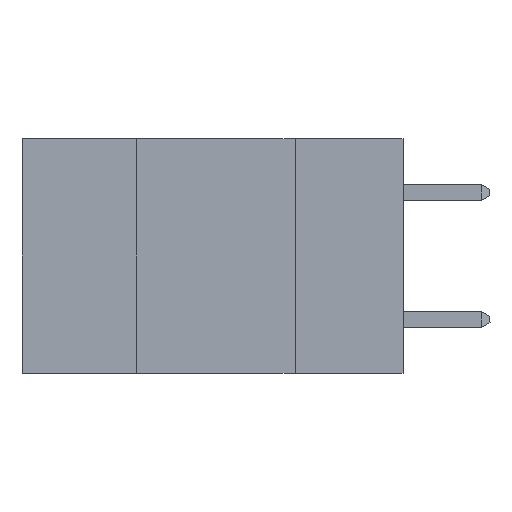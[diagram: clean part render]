
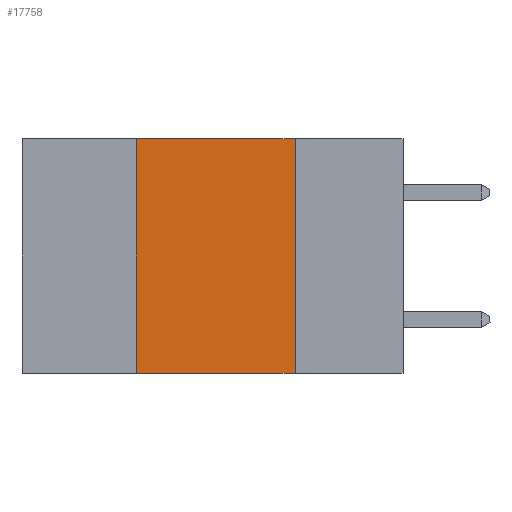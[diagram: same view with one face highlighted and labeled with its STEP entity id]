
A CAD part, left-side view. The second image highlights one B-rep face of the part: STEP entity #17758.
In plain terms, the highlighted planar face has unit normal (-1, 0, 0).
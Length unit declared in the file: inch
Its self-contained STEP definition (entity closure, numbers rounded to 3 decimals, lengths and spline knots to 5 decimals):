
#437 = CARTESIAN_POINT ( 'NONE',  ( 0., 0.42, 0. ) ) ;
#474 = VECTOR ( 'NONE', #4233, 39.37008 ) ;
#897 = EDGE_CURVE ( 'NONE', #2462, #2623, #10034, .T. ) ;
#1927 = DIRECTION ( 'NONE',  ( 0., 0., 1. ) ) ;
#2375 = VECTOR ( 'NONE', #11237, 39.37008 ) ;
#2462 = VERTEX_POINT ( 'NONE', #12152 ) ;
#2623 = VERTEX_POINT ( 'NONE', #8123 ) ;
#3463 = VERTEX_POINT ( 'NONE', #12853 ) ;
#3555 = LINE ( 'NONE', #18404, #474 ) ;
#4233 = DIRECTION ( 'NONE',  ( 0., -1., 0. ) ) ;
#4282 = DIRECTION ( 'NONE',  ( 1., 0., 0. ) ) ;
#4333 = EDGE_CURVE ( 'NONE', #3463, #2462, #12595, .T. ) ;
#5644 = PLANE ( 'NONE',  #18046 ) ;
#7131 = EDGE_CURVE ( 'NONE', #11442, #3463, #16711, .T. ) ;
#7782 = FACE_OUTER_BOUND ( 'NONE', #8943, .T. ) ;
#8123 = CARTESIAN_POINT ( 'NONE',  ( 0., 0.17, -0.37 ) ) ;
#8516 = VECTOR ( 'NONE', #1927, 39.37008 ) ;
#8943 = EDGE_LOOP ( 'NONE', ( #9367, #10799, #10862, #11374 ) ) ;
#9367 = ORIENTED_EDGE ( 'NONE', *, *, #897, .F. ) ;
#9485 = CARTESIAN_POINT ( 'NONE',  ( 0., 0.42, -0.37 ) ) ;
#10034 = LINE ( 'NONE', #13470, #2375 ) ;
#10799 = ORIENTED_EDGE ( 'NONE', *, *, #4333, .F. ) ;
#10862 = ORIENTED_EDGE ( 'NONE', *, *, #7131, .F. ) ;
#11237 = DIRECTION ( 'NONE',  ( 0., 0., -1. ) ) ;
#11374 = ORIENTED_EDGE ( 'NONE', *, *, #17147, .T. ) ;
#11442 = VERTEX_POINT ( 'NONE', #9485 ) ;
#12152 = CARTESIAN_POINT ( 'NONE',  ( 0., 0.17, 0. ) ) ;
#12595 = LINE ( 'NONE', #13329, #15930 ) ;
#12853 = CARTESIAN_POINT ( 'NONE',  ( 0., 0.42, 0. ) ) ;
#12936 = CARTESIAN_POINT ( 'NONE',  ( 0., 0.6, 0. ) ) ;
#13329 = CARTESIAN_POINT ( 'NONE',  ( 0., 0.6, 0. ) ) ;
#13470 = CARTESIAN_POINT ( 'NONE',  ( 0., 0.17, 0. ) ) ;
#14354 = DIRECTION ( 'NONE',  ( 0., 0., -1. ) ) ;
#14733 = DIRECTION ( 'NONE',  ( 0., -1., 0. ) ) ;
#15930 = VECTOR ( 'NONE', #14733, 39.37008 ) ;
#16711 = LINE ( 'NONE', #437, #8516 ) ;
#17147 = EDGE_CURVE ( 'NONE', #11442, #2623, #3555, .T. ) ;
#17758 = ADVANCED_FACE ( 'NONE', ( #7782 ), #5644, .F. ) ;
#18046 = AXIS2_PLACEMENT_3D ( 'NONE', #12936, #4282, #14354 ) ;
#18404 = CARTESIAN_POINT ( 'NONE',  ( 0., 0.6, -0.37 ) ) ;
